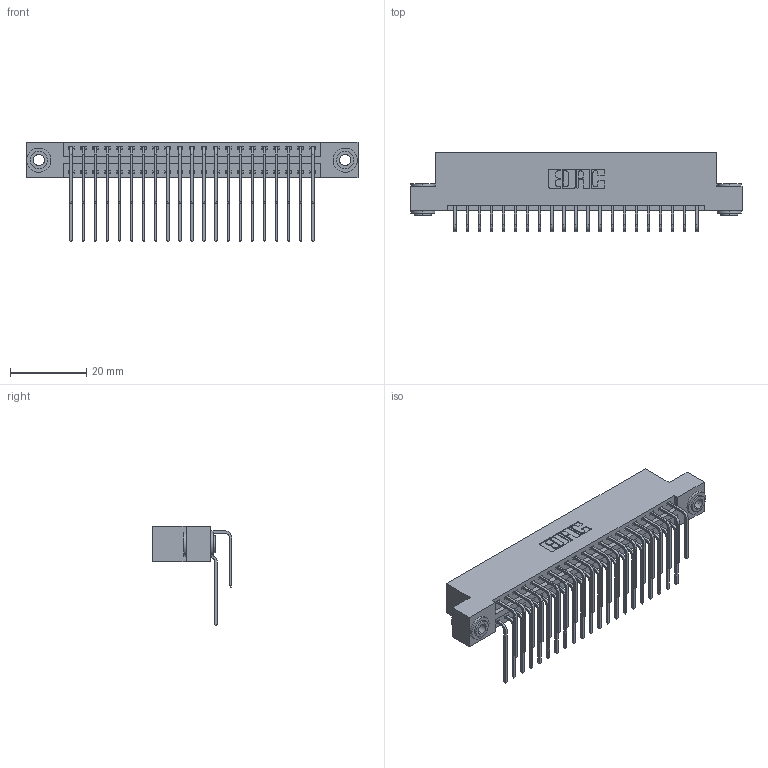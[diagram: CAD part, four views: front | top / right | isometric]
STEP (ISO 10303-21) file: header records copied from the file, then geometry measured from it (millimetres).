
FILE_DESCRIPTION (( 'STEP AP203' ), '1' );
FILE_NAME ('396-042-559-203.STEP', '2018-09-07T01:28:50', ( '' ), ( '' ), 'SwSTEP 2.0', 'SolidWorks 2016', '' );
FILE_SCHEMA (( 'CONFIG_CONTROL_DESIGN' ));
Length unit declared in the file: inch
Products named in the file (5): 345-250-002_345-250-002-102; 396-042-559-203; 346 Part_Flush Mounting Lugs - 0.156 Dia-TH; 345-292-001_558 559 Tail - 1; 345-292-001_559 Tail - 2
Assembly tree (45 placements, depth 2):
  396-042-559-203
    346 Part_Flush Mounting Lugs - 0.156 Dia-TH
    345-292-001_558 559 Tail - 1  x21
    345-292-001_559 Tail - 2  x21
    345-250-002_345-250-002-102  x2
Bounding box: 87.25 x 20.89 x 26.16 mm (x, y, z)
Volume: 8606.4 mm3; surface area: 12876.6 mm2
Topology: 45 solids, 45 shells, 2428 faces, 7167 edges, 4718 vertices
Faces by surface type: plane 1640, cylinder 780, cone 8
Entity records: 18966 total; most frequent: CARTESIAN_POINT 3182, ORIENTED_EDGE 3058, DIRECTION 2859, EDGE_CURVE 1529, LINE 1249, VECTOR 1249, VERTEX_POINT 1014, AXIS2_PLACEMENT_3D 805
